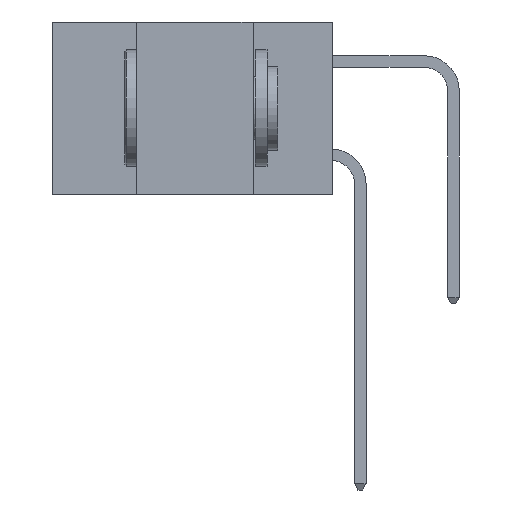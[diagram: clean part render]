
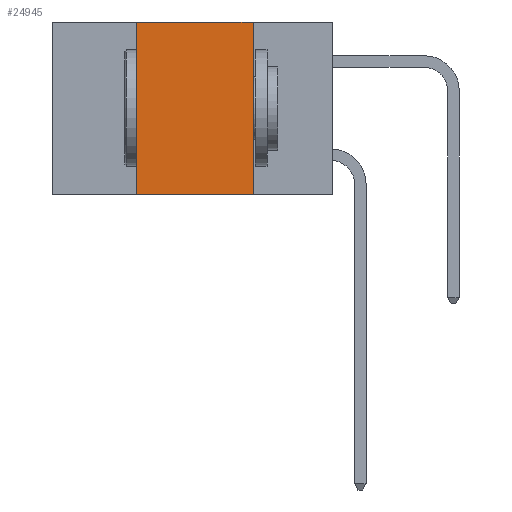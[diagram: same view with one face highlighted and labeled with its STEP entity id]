
A CAD part, left-side view. The second image highlights one B-rep face of the part: STEP entity #24945.
In plain terms, the highlighted planar face has unit normal (-1, 0, 0).
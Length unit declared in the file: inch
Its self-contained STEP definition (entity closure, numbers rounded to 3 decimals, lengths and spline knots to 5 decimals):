
#1023 = EDGE_LOOP ( 'NONE', ( #16830, #17524, #1238, #14471 ) ) ;
#1238 = ORIENTED_EDGE ( 'NONE', *, *, #15546, .F. ) ;
#2091 = DIRECTION ( 'NONE',  ( 0., 0., -1. ) ) ;
#2773 = PLANE ( 'NONE',  #3954 ) ;
#3248 = VERTEX_POINT ( 'NONE', #18641 ) ;
#3743 = CARTESIAN_POINT ( 'NONE',  ( 0., 0.6, -0.37 ) ) ;
#3954 = AXIS2_PLACEMENT_3D ( 'NONE', #18205, #5058, #20418 ) ;
#5058 = DIRECTION ( 'NONE',  ( 1., 0., 0. ) ) ;
#6486 = VECTOR ( 'NONE', #22040, 39.37008 ) ;
#6820 = EDGE_CURVE ( 'NONE', #15628, #3248, #15310, .T. ) ;
#7994 = EDGE_CURVE ( 'NONE', #12358, #17846, #18619, .T. ) ;
#8146 = CARTESIAN_POINT ( 'NONE',  ( 0., 0.6, 0. ) ) ;
#10246 = VECTOR ( 'NONE', #23604, 39.37008 ) ;
#12358 = VERTEX_POINT ( 'NONE', #17922 ) ;
#13563 = VECTOR ( 'NONE', #25685, 39.37008 ) ;
#14471 = ORIENTED_EDGE ( 'NONE', *, *, #6820, .T. ) ;
#15310 = LINE ( 'NONE', #3743, #10246 ) ;
#15546 = EDGE_CURVE ( 'NONE', #15628, #12358, #18120, .T. ) ;
#15628 = VERTEX_POINT ( 'NONE', #15719 ) ;
#15719 = CARTESIAN_POINT ( 'NONE',  ( 0., 0.42, -0.37 ) ) ;
#16766 = EDGE_CURVE ( 'NONE', #17846, #3248, #20107, .T. ) ;
#16830 = ORIENTED_EDGE ( 'NONE', *, *, #16766, .F. ) ;
#17524 = ORIENTED_EDGE ( 'NONE', *, *, #7994, .F. ) ;
#17846 = VERTEX_POINT ( 'NONE', #21347 ) ;
#17922 = CARTESIAN_POINT ( 'NONE',  ( 0., 0.42, 0. ) ) ;
#18120 = LINE ( 'NONE', #19811, #6486 ) ;
#18205 = CARTESIAN_POINT ( 'NONE',  ( 0., 0.6, 0. ) ) ;
#18619 = LINE ( 'NONE', #8146, #13563 ) ;
#18641 = CARTESIAN_POINT ( 'NONE',  ( 0., 0.17, -0.37 ) ) ;
#19811 = CARTESIAN_POINT ( 'NONE',  ( 0., 0.42, -0.37 ) ) ;
#20107 = LINE ( 'NONE', #24107, #25313 ) ;
#20418 = DIRECTION ( 'NONE',  ( 0., 0., -1. ) ) ;
#21347 = CARTESIAN_POINT ( 'NONE',  ( 0., 0.17, 0. ) ) ;
#22040 = DIRECTION ( 'NONE',  ( 0., 0., 1. ) ) ;
#23604 = DIRECTION ( 'NONE',  ( 0., -1., 0. ) ) ;
#24107 = CARTESIAN_POINT ( 'NONE',  ( 0., 0.17, -0.37 ) ) ;
#24945 = ADVANCED_FACE ( 'NONE', ( #27560 ), #2773, .F. ) ;
#25313 = VECTOR ( 'NONE', #2091, 39.37008 ) ;
#25685 = DIRECTION ( 'NONE',  ( 0., -1., 0. ) ) ;
#27560 = FACE_OUTER_BOUND ( 'NONE', #1023, .T. ) ;
